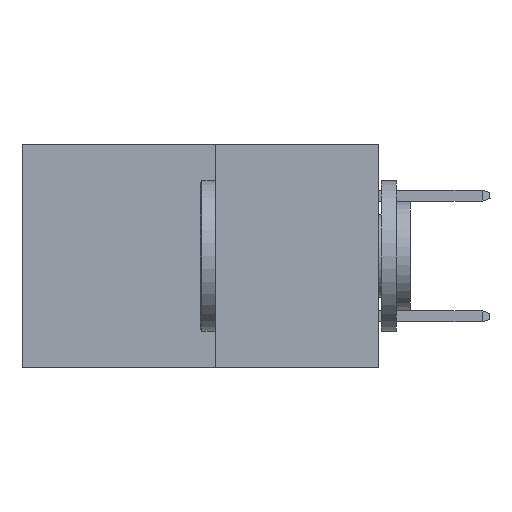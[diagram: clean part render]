
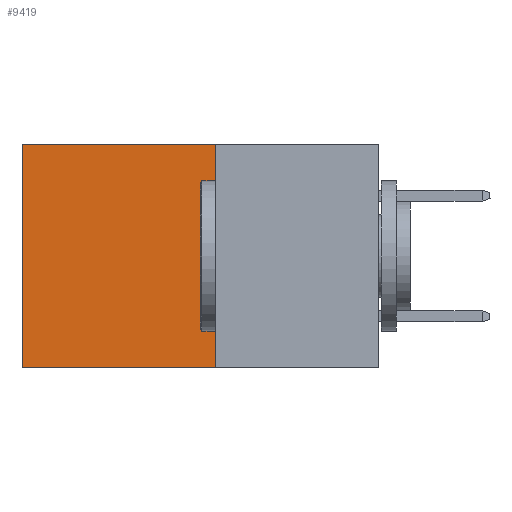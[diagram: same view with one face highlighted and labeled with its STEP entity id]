
A CAD part, left-side view. The second image highlights one B-rep face of the part: STEP entity #9419.
In plain terms, the highlighted planar face has unit normal (-1, 0, 0).
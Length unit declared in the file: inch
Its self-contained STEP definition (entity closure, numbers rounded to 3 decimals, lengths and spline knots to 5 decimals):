
#1128 = DIRECTION ( 'NONE',  ( 0., 1., 0. ) ) ;
#1544 = AXIS2_PLACEMENT_3D ( 'NONE', #24666, #27344, #11407 ) ;
#2100 = VERTEX_POINT ( 'NONE', #26232 ) ;
#3472 = EDGE_CURVE ( 'NONE', #2100, #11042, #22914, .T. ) ;
#4133 = EDGE_LOOP ( 'NONE', ( #22932, #17457, #13656, #13085 ) ) ;
#8833 = VECTOR ( 'NONE', #8974, 39.37008 ) ;
#8974 = DIRECTION ( 'NONE',  ( 0., 0., -1. ) ) ;
#9129 = CARTESIAN_POINT ( 'NONE',  ( 0.277, 0.27, -0.37 ) ) ;
#9368 = VERTEX_POINT ( 'NONE', #27105 ) ;
#9419 = ADVANCED_FACE ( 'NONE', ( #31451 ), #22000, .F. ) ;
#10008 = LINE ( 'NONE', #14948, #24129 ) ;
#10320 = VERTEX_POINT ( 'NONE', #17776 ) ;
#11042 = VERTEX_POINT ( 'NONE', #15286 ) ;
#11407 = DIRECTION ( 'NONE',  ( 0., 0., -1. ) ) ;
#11590 = EDGE_CURVE ( 'NONE', #2100, #10320, #32934, .T. ) ;
#11796 = VECTOR ( 'NONE', #1128, 39.37008 ) ;
#13085 = ORIENTED_EDGE ( 'NONE', *, *, #11590, .T. ) ;
#13656 = ORIENTED_EDGE ( 'NONE', *, *, #3472, .F. ) ;
#14948 = CARTESIAN_POINT ( 'NONE',  ( 0.277, 0.59, -0.37 ) ) ;
#15286 = CARTESIAN_POINT ( 'NONE',  ( 0.277, 0.27, -0.37 ) ) ;
#16496 = EDGE_CURVE ( 'NONE', #11042, #9368, #19643, .T. ) ;
#17444 = EDGE_CURVE ( 'NONE', #10320, #9368, #10008, .T. ) ;
#17457 = ORIENTED_EDGE ( 'NONE', *, *, #16496, .F. ) ;
#17776 = CARTESIAN_POINT ( 'NONE',  ( 0.277, 0.59, 0. ) ) ;
#19643 = LINE ( 'NONE', #29749, #32857 ) ;
#22000 = PLANE ( 'NONE',  #1544 ) ;
#22914 = LINE ( 'NONE', #9129, #8833 ) ;
#22932 = ORIENTED_EDGE ( 'NONE', *, *, #17444, .T. ) ;
#24129 = VECTOR ( 'NONE', #33465, 39.37008 ) ;
#24666 = CARTESIAN_POINT ( 'NONE',  ( 0.277, 0.27, -0.37 ) ) ;
#26232 = CARTESIAN_POINT ( 'NONE',  ( 0.277, 0.27, 0. ) ) ;
#27092 = DIRECTION ( 'NONE',  ( 0., 1., 0. ) ) ;
#27105 = CARTESIAN_POINT ( 'NONE',  ( 0.277, 0.59, -0.37 ) ) ;
#27344 = DIRECTION ( 'NONE',  ( 1., 0., 0. ) ) ;
#29749 = CARTESIAN_POINT ( 'NONE',  ( 0.277, 0.27, -0.37 ) ) ;
#31451 = FACE_OUTER_BOUND ( 'NONE', #4133, .T. ) ;
#32857 = VECTOR ( 'NONE', #27092, 39.37008 ) ;
#32898 = CARTESIAN_POINT ( 'NONE',  ( 0.277, 0.27, 0. ) ) ;
#32934 = LINE ( 'NONE', #32898, #11796 ) ;
#33465 = DIRECTION ( 'NONE',  ( 0., 0., -1. ) ) ;
